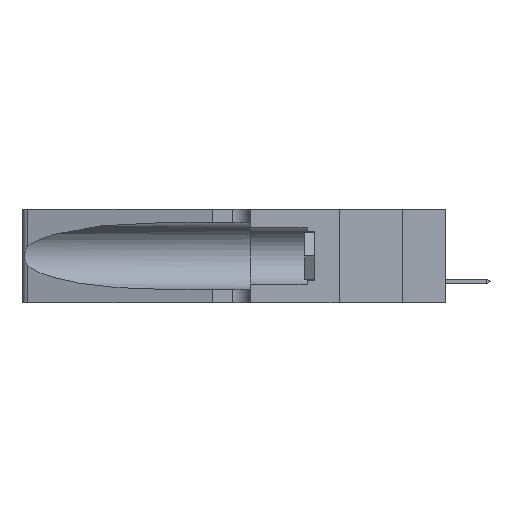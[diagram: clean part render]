
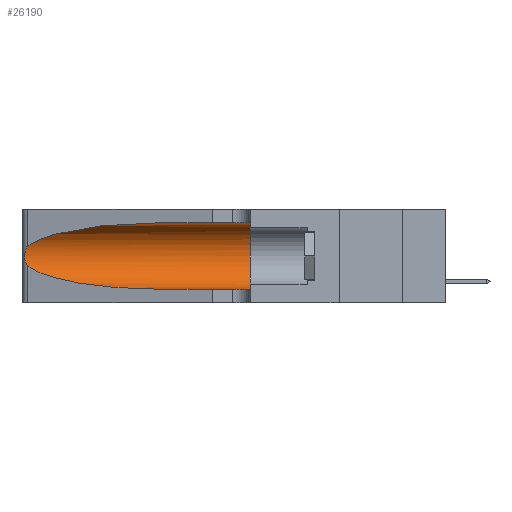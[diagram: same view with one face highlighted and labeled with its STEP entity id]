
A CAD part, left-side view. The second image highlights one B-rep face of the part: STEP entity #26190.
In plain terms, the highlighted cylindrical face has radius 3.308 mm (diameter 6.617 mm), a partial arc.
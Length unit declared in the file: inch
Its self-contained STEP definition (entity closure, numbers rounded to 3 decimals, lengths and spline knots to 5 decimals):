
#1264 = VERTEX_POINT ( 'NONE', #28628 ) ;
#2092 = VERTEX_POINT ( 'NONE', #20091 ) ;
#2723 = CARTESIAN_POINT ( 'NONE',  ( 0.1305, 0.72297, 0.05475 ) ) ;
#2837 = CARTESIAN_POINT ( 'NONE',  ( 0.26018, 1.23835, 0.19895 ) ) ;
#2997 = CARTESIAN_POINT ( 'NONE',  ( 0.26075, 1.23896, 0.178 ) ) ;
#3012 = LINE ( 'NONE', #8306, #28171 ) ;
#4270 = DIRECTION ( 'NONE',  ( 0., -1., 0. ) ) ;
#4950 = ORIENTED_EDGE ( 'NONE', *, *, #28529, .T. ) ;
#6735 = CARTESIAN_POINT ( 'NONE',  ( 0.26075, 1.23896, 0.19203 ) ) ;
#6821 = EDGE_CURVE ( 'NONE', #8292, #42368, #23288, .T. ) ;
#7257 = CARTESIAN_POINT ( 'NONE',  ( 0.2373, 1.15595, 0.28018 ) ) ;
#8292 = VERTEX_POINT ( 'NONE', #13580 ) ;
#8306 = CARTESIAN_POINT ( 'NONE',  ( 0.1305, 1.61858, 0.05475 ) ) ;
#9892 = CARTESIAN_POINT ( 'NONE',  ( 0.25487, 1.22718, 0.14631 ) ) ;
#11336 = AXIS2_PLACEMENT_3D ( 'NONE', #34779, #31436, #31720 ) ;
#12653 = EDGE_CURVE ( 'NONE', #31630, #8292, #26593, .T. ) ;
#12793 = EDGE_LOOP ( 'NONE', ( #4950, #24853, #32354, #15911, #42682, #17146 ) ) ;
#12806 = FACE_OUTER_BOUND ( 'NONE', #12793, .T. ) ;
#12908 = DIRECTION ( 'NONE',  ( 0., -1., 0. ) ) ;
#13202 = CARTESIAN_POINT ( 'NONE',  ( 0.25555, 1.22993, 0.14849 ) ) ;
#13467 = CARTESIAN_POINT ( 'NONE',  ( 0.2373, 1.15595, 0.08982 ) ) ;
#13580 = CARTESIAN_POINT ( 'NONE',  ( 0.25487, 1.22718, 0.14631 ) ) ;
#15911 = ORIENTED_EDGE ( 'NONE', *, *, #22912, .T. ) ;
#17146 = ORIENTED_EDGE ( 'NONE', *, *, #35305, .F. ) ;
#17226 = CARTESIAN_POINT ( 'NONE',  ( 0.18966, 0.96281, 0.05475 ) ) ;
#19954 = CARTESIAN_POINT ( 'NONE',  ( 0.25555, 1.22994, 0.2215 ) ) ;
#20091 = CARTESIAN_POINT ( 'NONE',  ( 0.1305, 0.72297, 0.31525 ) ) ;
#21651 = AXIS2_PLACEMENT_3D ( 'NONE', #27312, #12908, #40475 ) ;
#22912 = EDGE_CURVE ( 'NONE', #42368, #36315, #3012, .T. ) ;
#23288 =( BOUNDED_CURVE ( )  B_SPLINE_CURVE ( 3, ( #9892, #13467, #17226, #24099 ),
 .UNSPECIFIED., .F., .T. ) 
 B_SPLINE_CURVE_WITH_KNOTS ( ( 4, 4 ),
 ( 3.44316, 4.71239 ),
 .UNSPECIFIED. ) 
 CURVE ( )  GEOMETRIC_REPRESENTATION_ITEM ( )  RATIONAL_B_SPLINE_CURVE ( ( 1., 0.87, 0.87, 1. ) ) 
 REPRESENTATION_ITEM ( '' )  );
#23429 = CARTESIAN_POINT ( 'NONE',  ( 0.25854, 1.2359, 0.20912 ) ) ;
#23488 = VECTOR ( 'NONE', #4270, 39.37008 ) ;
#23846 =( BOUNDED_CURVE ( )  B_SPLINE_CURVE ( 3, ( #44160, #41439, #7257, #27950 ),
 .UNSPECIFIED., .F., .F. ) 
 B_SPLINE_CURVE_WITH_KNOTS ( ( 4, 4 ),
 ( 1.5708, 2.84003 ),
 .UNSPECIFIED. ) 
 CURVE ( )  GEOMETRIC_REPRESENTATION_ITEM ( )  RATIONAL_B_SPLINE_CURVE ( ( 1., 0.87, 0.87, 1. ) ) 
 REPRESENTATION_ITEM ( '' )  );
#24099 = CARTESIAN_POINT ( 'NONE',  ( 0.1305, 0.72297, 0.05475 ) ) ;
#24853 = ORIENTED_EDGE ( 'NONE', *, *, #12653, .T. ) ;
#25746 = CARTESIAN_POINT ( 'NONE',  ( 0.25487, 1.22718, 0.22369 ) ) ;
#26190 = ADVANCED_FACE ( 'NONE', ( #12806 ), #40860, .F. ) ;
#26593 = B_SPLINE_CURVE_WITH_KNOTS ( 'NONE', 3,
 ( #44015, #19954, #27166, #44179, #23429, #2837, #6735, #2997, #30611, #30321, #30759, #33793, #13202, #37265 ),
 .UNSPECIFIED., .F., .F.,
 ( 4, 2, 2, 2, 2, 2, 4 ),
 ( 0., 0.00027, 0.00053, 0.00107, 0.0016, 0.00187, 0.00214 ),
 .UNSPECIFIED. ) ;
#27166 = CARTESIAN_POINT ( 'NONE',  ( 0.25639, 1.23184, 0.21858 ) ) ;
#27197 = CARTESIAN_POINT ( 'NONE',  ( 0.1305, 0.35, 0.05475 ) ) ;
#27312 = CARTESIAN_POINT ( 'NONE',  ( 0.1305, 1.61858, 0.185 ) ) ;
#27950 = CARTESIAN_POINT ( 'NONE',  ( 0.25487, 1.22718, 0.22369 ) ) ;
#28171 = VECTOR ( 'NONE', #41276, 39.37008 ) ;
#28529 = EDGE_CURVE ( 'NONE', #2092, #31630, #23846, .T. ) ;
#28628 = CARTESIAN_POINT ( 'NONE',  ( 0.1305, 0.35, 0.31525 ) ) ;
#28765 = CARTESIAN_POINT ( 'NONE',  ( 0.1305, 1.61858, 0.31525 ) ) ;
#30321 = CARTESIAN_POINT ( 'NONE',  ( 0.25856, 1.23593, 0.16098 ) ) ;
#30611 = CARTESIAN_POINT ( 'NONE',  ( 0.26017, 1.23833, 0.17102 ) ) ;
#30759 = CARTESIAN_POINT ( 'NONE',  ( 0.25789, 1.23486, 0.15765 ) ) ;
#31436 = DIRECTION ( 'NONE',  ( 0., 1., 0. ) ) ;
#31630 = VERTEX_POINT ( 'NONE', #25746 ) ;
#31720 = DIRECTION ( 'NONE',  ( 0., 0., 1. ) ) ;
#32354 = ORIENTED_EDGE ( 'NONE', *, *, #6821, .T. ) ;
#33711 = LINE ( 'NONE', #28765, #23488 ) ;
#33793 = CARTESIAN_POINT ( 'NONE',  ( 0.25639, 1.23186, 0.15144 ) ) ;
#34076 = CIRCLE ( 'NONE', #11336, 0.13025 ) ;
#34779 = CARTESIAN_POINT ( 'NONE',  ( 0.1305, 0.35, 0.185 ) ) ;
#35305 = EDGE_CURVE ( 'NONE', #2092, #1264, #33711, .T. ) ;
#36315 = VERTEX_POINT ( 'NONE', #27197 ) ;
#37265 = CARTESIAN_POINT ( 'NONE',  ( 0.25487, 1.22718, 0.14631 ) ) ;
#40127 = EDGE_CURVE ( 'NONE', #1264, #36315, #34076, .T. ) ;
#40475 = DIRECTION ( 'NONE',  ( 0., 0., -1. ) ) ;
#40860 = CYLINDRICAL_SURFACE ( 'NONE', #21651, 0.13025 ) ;
#41276 = DIRECTION ( 'NONE',  ( 0., -1., 0. ) ) ;
#41439 = CARTESIAN_POINT ( 'NONE',  ( 0.18966, 0.96281, 0.31525 ) ) ;
#42368 = VERTEX_POINT ( 'NONE', #2723 ) ;
#42682 = ORIENTED_EDGE ( 'NONE', *, *, #40127, .F. ) ;
#44015 = CARTESIAN_POINT ( 'NONE',  ( 0.25487, 1.22718, 0.22369 ) ) ;
#44160 = CARTESIAN_POINT ( 'NONE',  ( 0.1305, 0.72297, 0.31525 ) ) ;
#44179 = CARTESIAN_POINT ( 'NONE',  ( 0.25787, 1.23484, 0.2124 ) ) ;
